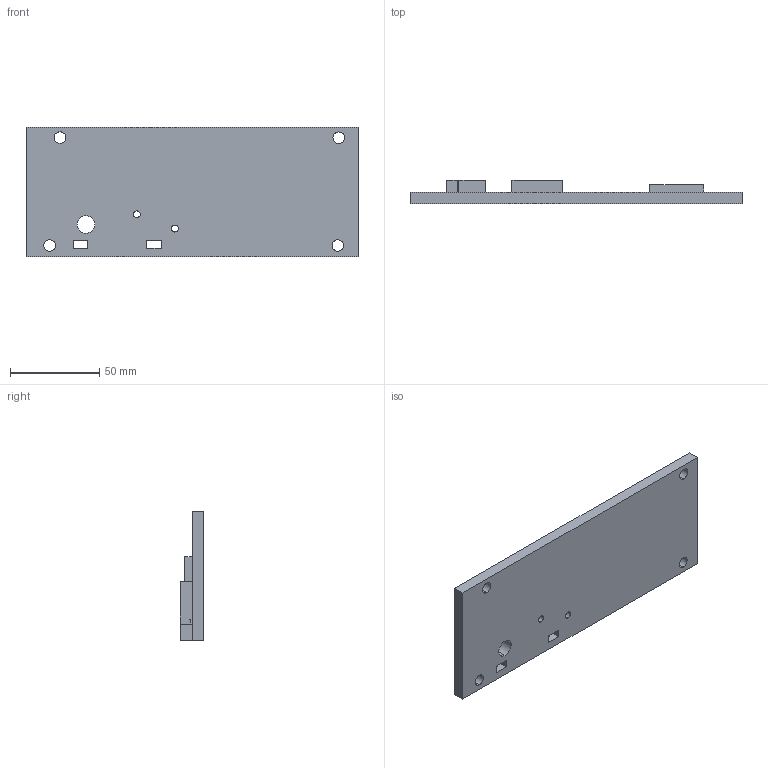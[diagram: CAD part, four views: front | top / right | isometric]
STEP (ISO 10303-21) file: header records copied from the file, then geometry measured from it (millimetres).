
FILE_DESCRIPTION (( 'STEP AP203' ), '1' );
FILE_NAME ('LeftSideWall.STEP', '2019-06-30T00:55:41', ( '' ), ( '' ), 'SwSTEP 2.0', 'SolidWorks 2017', '' );
FILE_SCHEMA (( 'CONFIG_CONTROL_DESIGN' ));
Length unit declared in the file: millimetre
Products named in the file (1): LeftSideWall
Bounding box: 186.5 x 13.3 x 73 mm (x, y, z)
Volume: 99754.5 mm3; surface area: 34385.9 mm2
Topology: 1 solids, 1 shells, 59 faces, 164 edges, 109 vertices
Faces by surface type: plane 36, cylinder 23
Entity records: 2017 total; most frequent: CARTESIAN_POINT 333, DIRECTION 330, ORIENTED_EDGE 328, EDGE_CURVE 164, LINE 118, VECTOR 118, VERTEX_POINT 109, AXIS2_PLACEMENT_3D 106
